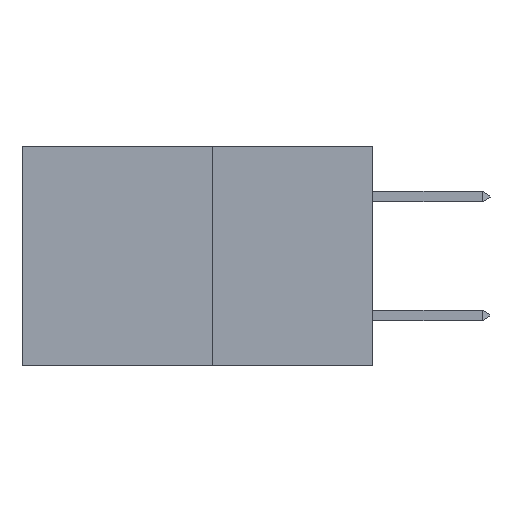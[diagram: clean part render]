
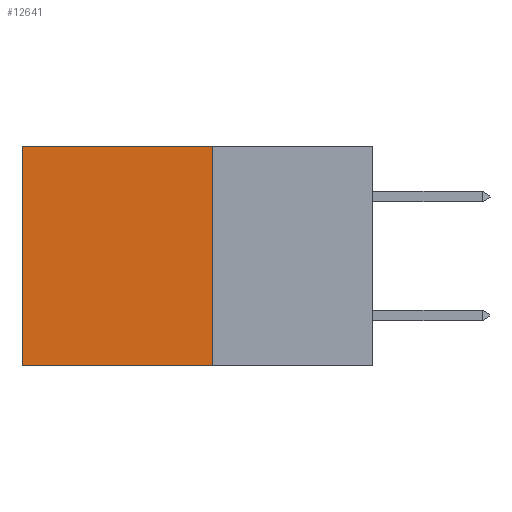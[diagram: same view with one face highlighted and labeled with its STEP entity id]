
A CAD part, left-side view. The second image highlights one B-rep face of the part: STEP entity #12641.
In plain terms, the highlighted planar face has unit normal (-1, 0, 0).
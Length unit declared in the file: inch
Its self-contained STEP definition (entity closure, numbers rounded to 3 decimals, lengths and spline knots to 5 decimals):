
#1406 = CARTESIAN_POINT ( 'NONE',  ( 0.277, 0.27, -0.37 ) ) ;
#2049 = FACE_OUTER_BOUND ( 'NONE', #7716, .T. ) ;
#2599 = PLANE ( 'NONE',  #9611 ) ;
#3003 = EDGE_CURVE ( 'NONE', #12158, #16262, #7641, .T. ) ;
#3017 = DIRECTION ( 'NONE',  ( 0., 0., -1. ) ) ;
#4195 = DIRECTION ( 'NONE',  ( 1., 0., 0. ) ) ;
#5121 = CARTESIAN_POINT ( 'NONE',  ( 0.277, 0.27, 0. ) ) ;
#5559 = EDGE_CURVE ( 'NONE', #7561, #6110, #18106, .T. ) ;
#6110 = VERTEX_POINT ( 'NONE', #19267 ) ;
#7148 = ORIENTED_EDGE ( 'NONE', *, *, #9661, .T. ) ;
#7561 = VERTEX_POINT ( 'NONE', #12293 ) ;
#7641 = LINE ( 'NONE', #1406, #19334 ) ;
#7652 = CARTESIAN_POINT ( 'NONE',  ( 0.277, 0.27, -0.37 ) ) ;
#7716 = EDGE_LOOP ( 'NONE', ( #18194, #17753, #16812, #7148 ) ) ;
#8708 = VECTOR ( 'NONE', #12491, 39.37008 ) ;
#9197 = LINE ( 'NONE', #17034, #8708 ) ;
#9611 = AXIS2_PLACEMENT_3D ( 'NONE', #13554, #4195, #15090 ) ;
#9661 = EDGE_CURVE ( 'NONE', #12158, #7561, #13674, .T. ) ;
#10418 = VECTOR ( 'NONE', #13387, 39.37008 ) ;
#12158 = VERTEX_POINT ( 'NONE', #12663 ) ;
#12293 = CARTESIAN_POINT ( 'NONE',  ( 0.277, 0.59, 0. ) ) ;
#12491 = DIRECTION ( 'NONE',  ( 0., 1., 0. ) ) ;
#12641 = ADVANCED_FACE ( 'NONE', ( #2049 ), #2599, .F. ) ;
#12663 = CARTESIAN_POINT ( 'NONE',  ( 0.277, 0.27, 0. ) ) ;
#13167 = VECTOR ( 'NONE', #17484, 39.37008 ) ;
#13387 = DIRECTION ( 'NONE',  ( 0., 0., -1. ) ) ;
#13554 = CARTESIAN_POINT ( 'NONE',  ( 0.277, 0.27, -0.37 ) ) ;
#13580 = EDGE_CURVE ( 'NONE', #16262, #6110, #9197, .T. ) ;
#13674 = LINE ( 'NONE', #5121, #13167 ) ;
#15090 = DIRECTION ( 'NONE',  ( 0., 0., -1. ) ) ;
#16262 = VERTEX_POINT ( 'NONE', #7652 ) ;
#16444 = CARTESIAN_POINT ( 'NONE',  ( 0.277, 0.59, -0.37 ) ) ;
#16812 = ORIENTED_EDGE ( 'NONE', *, *, #3003, .F. ) ;
#17034 = CARTESIAN_POINT ( 'NONE',  ( 0.277, 0.27, -0.37 ) ) ;
#17484 = DIRECTION ( 'NONE',  ( 0., 1., 0. ) ) ;
#17753 = ORIENTED_EDGE ( 'NONE', *, *, #13580, .F. ) ;
#18106 = LINE ( 'NONE', #16444, #10418 ) ;
#18194 = ORIENTED_EDGE ( 'NONE', *, *, #5559, .T. ) ;
#19267 = CARTESIAN_POINT ( 'NONE',  ( 0.277, 0.59, -0.37 ) ) ;
#19334 = VECTOR ( 'NONE', #3017, 39.37008 ) ;
